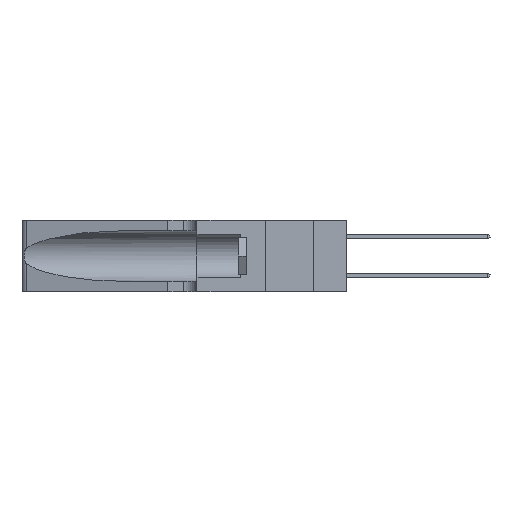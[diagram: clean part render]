
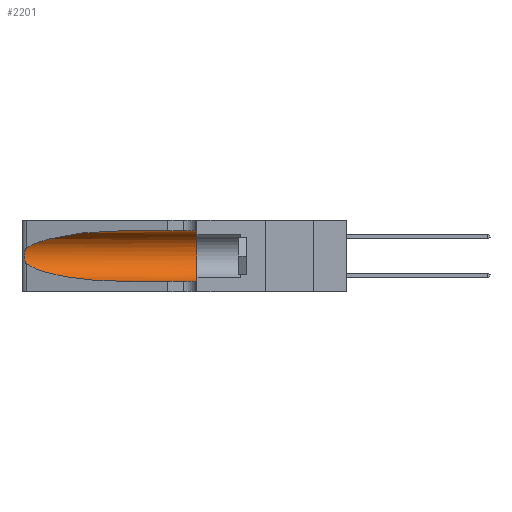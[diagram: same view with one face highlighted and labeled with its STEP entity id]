
A CAD part, left-side view. The second image highlights one B-rep face of the part: STEP entity #2201.
In plain terms, the highlighted cylindrical face has radius 3.308 mm (diameter 6.617 mm), a partial arc.
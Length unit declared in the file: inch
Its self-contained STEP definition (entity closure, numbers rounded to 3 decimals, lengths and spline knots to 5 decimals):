
#504 = CARTESIAN_POINT ( 'NONE',  ( 0.25856, 1.23593, 0.16098 ) ) ;
#682 = AXIS2_PLACEMENT_3D ( 'NONE', #17189, #9498, #3765 ) ;
#773 = VECTOR ( 'NONE', #15929, 39.37008 ) ;
#980 = EDGE_CURVE ( 'NONE', #18648, #8194, #8415, .T. ) ;
#1253 = VERTEX_POINT ( 'NONE', #23896 ) ;
#1587 = EDGE_CURVE ( 'NONE', #6177, #13545, #8711, .T. ) ;
#1992 = DIRECTION ( 'NONE',  ( 0., -1., 0. ) ) ;
#2201 = ADVANCED_FACE ( 'NONE', ( #24005 ), #16181, .F. ) ;
#2552 = CARTESIAN_POINT ( 'NONE',  ( 0.26017, 1.23833, 0.17102 ) ) ;
#2944 = EDGE_LOOP ( 'NONE', ( #24341, #23961, #22396, #3879, #24833, #3662 ) ) ;
#3662 = ORIENTED_EDGE ( 'NONE', *, *, #7110, .F. ) ;
#3765 = DIRECTION ( 'NONE',  ( 0., 0., 1. ) ) ;
#3879 = ORIENTED_EDGE ( 'NONE', *, *, #6764, .T. ) ;
#4038 = EDGE_CURVE ( 'NONE', #13545, #1253, #22871, .T. ) ;
#4260 = CARTESIAN_POINT ( 'NONE',  ( 0.25487, 1.22718, 0.22369 ) ) ;
#4677 = EDGE_CURVE ( 'NONE', #1253, #23973, #10982, .T. ) ;
#4823 = CARTESIAN_POINT ( 'NONE',  ( 0.2373, 1.15595, 0.28018 ) ) ;
#4897 = CARTESIAN_POINT ( 'NONE',  ( 0.2373, 1.15595, 0.08982 ) ) ;
#5118 = CARTESIAN_POINT ( 'NONE',  ( 0.25487, 1.22718, 0.14631 ) ) ;
#5382 = CARTESIAN_POINT ( 'NONE',  ( 0.1305, 0.35, 0.05475 ) ) ;
#5884 = LINE ( 'NONE', #6382, #773 ) ;
#6177 = VERTEX_POINT ( 'NONE', #8168 ) ;
#6382 = CARTESIAN_POINT ( 'NONE',  ( 0.1305, 1.61858, 0.05475 ) ) ;
#6487 = CARTESIAN_POINT ( 'NONE',  ( 0.25854, 1.2359, 0.20912 ) ) ;
#6764 = EDGE_CURVE ( 'NONE', #23973, #8194, #5884, .T. ) ;
#7110 = EDGE_CURVE ( 'NONE', #6177, #18648, #12491, .T. ) ;
#8168 = CARTESIAN_POINT ( 'NONE',  ( 0.1305, 0.72297, 0.31525 ) ) ;
#8194 = VERTEX_POINT ( 'NONE', #5382 ) ;
#8415 = CIRCLE ( 'NONE', #682, 0.13025 ) ;
#8469 = CARTESIAN_POINT ( 'NONE',  ( 0.25487, 1.22718, 0.22369 ) ) ;
#8535 = CARTESIAN_POINT ( 'NONE',  ( 0.1305, 1.61858, 0.185 ) ) ;
#8711 =( BOUNDED_CURVE ( )  B_SPLINE_CURVE ( 3, ( #14211, #18529, #4823, #8469 ),
 .UNSPECIFIED., .F., .T. ) 
 B_SPLINE_CURVE_WITH_KNOTS ( ( 4, 4 ),
 ( 1.5708, 2.84003 ),
 .UNSPECIFIED. ) 
 CURVE ( )  GEOMETRIC_REPRESENTATION_ITEM ( )  RATIONAL_B_SPLINE_CURVE ( ( 1., 0.87, 0.87, 1. ) ) 
 REPRESENTATION_ITEM ( '' )  );
#8957 = CARTESIAN_POINT ( 'NONE',  ( 0.1305, 0.72297, 0.05475 ) ) ;
#9468 = CARTESIAN_POINT ( 'NONE',  ( 0.25555, 1.22994, 0.2215 ) ) ;
#9498 = DIRECTION ( 'NONE',  ( 0., 1., 0. ) ) ;
#10982 =( BOUNDED_CURVE ( )  B_SPLINE_CURVE ( 3, ( #5118, #4897, #18595, #8957 ),
 .UNSPECIFIED., .F., .F. ) 
 B_SPLINE_CURVE_WITH_KNOTS ( ( 4, 4 ),
 ( 3.44316, 4.71239 ),
 .UNSPECIFIED. ) 
 CURVE ( )  GEOMETRIC_REPRESENTATION_ITEM ( )  RATIONAL_B_SPLINE_CURVE ( ( 1., 0.87, 0.87, 1. ) ) 
 REPRESENTATION_ITEM ( '' )  );
#11979 = CARTESIAN_POINT ( 'NONE',  ( 0.26018, 1.23835, 0.19895 ) ) ;
#12491 = LINE ( 'NONE', #19215, #22111 ) ;
#13405 = AXIS2_PLACEMENT_3D ( 'NONE', #8535, #20222, #18336 ) ;
#13545 = VERTEX_POINT ( 'NONE', #4260 ) ;
#13959 = CARTESIAN_POINT ( 'NONE',  ( 0.25555, 1.22993, 0.14849 ) ) ;
#14211 = CARTESIAN_POINT ( 'NONE',  ( 0.1305, 0.72297, 0.31525 ) ) ;
#15786 = CARTESIAN_POINT ( 'NONE',  ( 0.26075, 1.23896, 0.178 ) ) ;
#15863 = CARTESIAN_POINT ( 'NONE',  ( 0.25787, 1.23484, 0.2124 ) ) ;
#15929 = DIRECTION ( 'NONE',  ( 0., -1., 0. ) ) ;
#16112 = CARTESIAN_POINT ( 'NONE',  ( 0.1305, 0.35, 0.31525 ) ) ;
#16181 = CYLINDRICAL_SURFACE ( 'NONE', #13405, 0.13025 ) ;
#17189 = CARTESIAN_POINT ( 'NONE',  ( 0.1305, 0.35, 0.185 ) ) ;
#17263 = CARTESIAN_POINT ( 'NONE',  ( 0.1305, 0.72297, 0.05475 ) ) ;
#17407 = CARTESIAN_POINT ( 'NONE',  ( 0.25487, 1.22718, 0.22369 ) ) ;
#17836 = CARTESIAN_POINT ( 'NONE',  ( 0.25487, 1.22718, 0.14631 ) ) ;
#18336 = DIRECTION ( 'NONE',  ( 0., 0., -1. ) ) ;
#18529 = CARTESIAN_POINT ( 'NONE',  ( 0.18966, 0.96281, 0.31525 ) ) ;
#18595 = CARTESIAN_POINT ( 'NONE',  ( 0.18966, 0.96281, 0.05475 ) ) ;
#18648 = VERTEX_POINT ( 'NONE', #16112 ) ;
#19215 = CARTESIAN_POINT ( 'NONE',  ( 0.1305, 1.61858, 0.31525 ) ) ;
#19671 = CARTESIAN_POINT ( 'NONE',  ( 0.25789, 1.23486, 0.15765 ) ) ;
#19751 = CARTESIAN_POINT ( 'NONE',  ( 0.26075, 1.23896, 0.19203 ) ) ;
#20222 = DIRECTION ( 'NONE',  ( 0., -1., 0. ) ) ;
#21734 = CARTESIAN_POINT ( 'NONE',  ( 0.25639, 1.23186, 0.15144 ) ) ;
#22111 = VECTOR ( 'NONE', #1992, 39.37008 ) ;
#22396 = ORIENTED_EDGE ( 'NONE', *, *, #4677, .T. ) ;
#22871 = B_SPLINE_CURVE_WITH_KNOTS ( 'NONE', 3,
 ( #17407, #9468, #23517, #15863, #6487, #11979, #19751, #15786, #2552, #504, #19671, #21734, #13959, #17836 ),
 .UNSPECIFIED., .F., .F.,
 ( 4, 2, 2, 2, 2, 2, 4 ),
 ( 0., 0.00027, 0.00053, 0.00107, 0.0016, 0.00187, 0.00214 ),
 .UNSPECIFIED. ) ;
#23517 = CARTESIAN_POINT ( 'NONE',  ( 0.25639, 1.23184, 0.21858 ) ) ;
#23896 = CARTESIAN_POINT ( 'NONE',  ( 0.25487, 1.22718, 0.14631 ) ) ;
#23961 = ORIENTED_EDGE ( 'NONE', *, *, #4038, .T. ) ;
#23973 = VERTEX_POINT ( 'NONE', #17263 ) ;
#24005 = FACE_OUTER_BOUND ( 'NONE', #2944, .T. ) ;
#24341 = ORIENTED_EDGE ( 'NONE', *, *, #1587, .T. ) ;
#24833 = ORIENTED_EDGE ( 'NONE', *, *, #980, .F. ) ;
